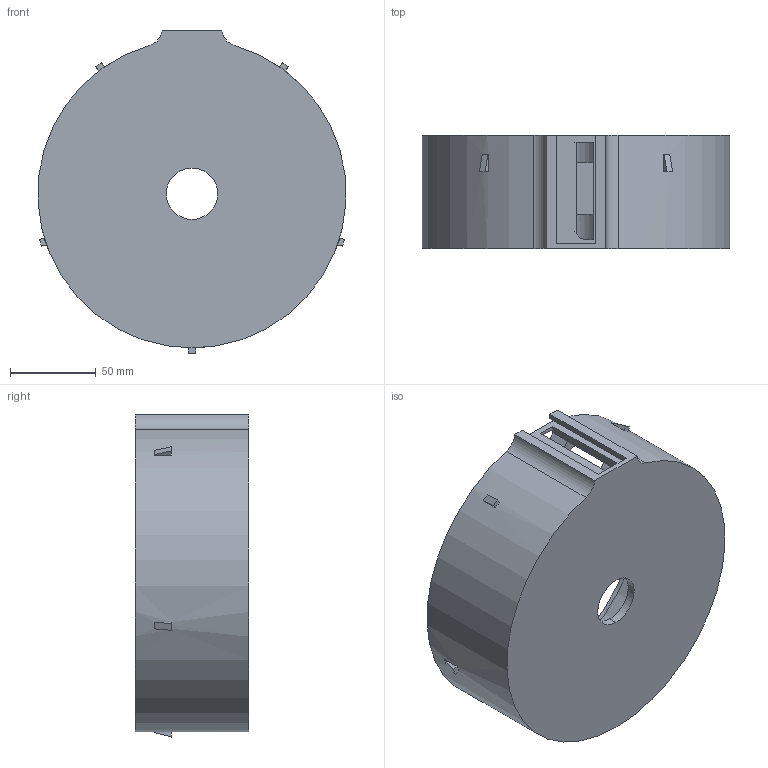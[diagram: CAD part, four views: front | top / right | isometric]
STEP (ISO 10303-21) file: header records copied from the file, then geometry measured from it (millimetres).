
FILE_DESCRIPTION (( 'STEP AP214' ), '1' );
FILE_NAME ('front.STEP', '2013-12-22T02:39:04', ( '' ), ( '' ), 'SwSTEP 2.0', 'SolidWorks 2013', '' );
FILE_SCHEMA (( 'AUTOMOTIVE_DESIGN' ));
Length unit declared in the file: millimetre
Products named in the file (1): front
Bounding box: 179.73 x 66 x 188 mm (x, y, z)
Volume: 353640.5 mm3; surface area: 152533.1 mm2
Topology: 1 solids, 1 shells, 97 faces, 259 edges, 168 vertices
Faces by surface type: plane 48, cylinder 33, torus 16
Entity records: 3330 total; most frequent: CARTESIAN_POINT 797, DIRECTION 548, ORIENTED_EDGE 518, EDGE_CURVE 259, AXIS2_PLACEMENT_3D 209, VERTEX_POINT 168, VECTOR 130, LINE 130
